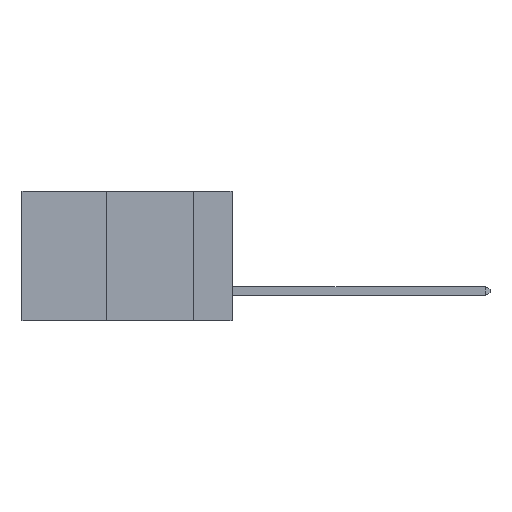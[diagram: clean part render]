
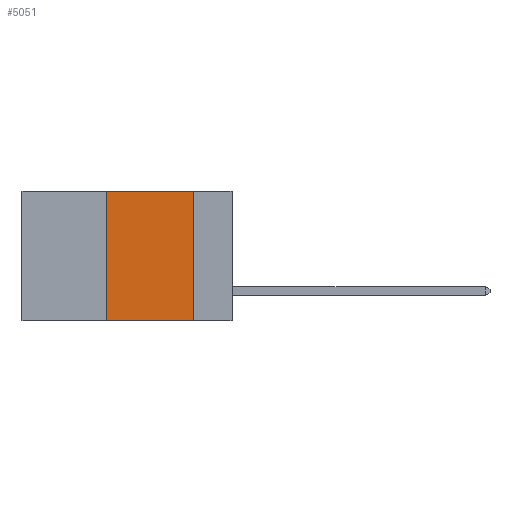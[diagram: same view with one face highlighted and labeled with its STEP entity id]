
A CAD part, left-side view. The second image highlights one B-rep face of the part: STEP entity #5051.
In plain terms, the highlighted planar face has unit normal (-1, 0, 0).
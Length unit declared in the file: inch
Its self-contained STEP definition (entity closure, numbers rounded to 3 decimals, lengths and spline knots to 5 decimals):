
#315 = ORIENTED_EDGE ( 'NONE', *, *, #6782, .F. ) ;
#455 = VECTOR ( 'NONE', #13491, 39.37008 ) ;
#505 = ORIENTED_EDGE ( 'NONE', *, *, #12875, .T. ) ;
#1597 = CARTESIAN_POINT ( 'NONE',  ( 0., 0.11, 0. ) ) ;
#2081 = CARTESIAN_POINT ( 'NONE',  ( 0., 0.6, 0. ) ) ;
#2132 = DIRECTION ( 'NONE',  ( 0., -1., 0. ) ) ;
#2200 = EDGE_CURVE ( 'NONE', #9139, #2787, #4364, .T. ) ;
#2245 = ORIENTED_EDGE ( 'NONE', *, *, #2200, .F. ) ;
#2416 = DIRECTION ( 'NONE',  ( 0., 0., 1. ) ) ;
#2787 = VERTEX_POINT ( 'NONE', #1597 ) ;
#3052 = CARTESIAN_POINT ( 'NONE',  ( 0., 0.6, 0. ) ) ;
#3167 = CARTESIAN_POINT ( 'NONE',  ( 0., 0.36, 0. ) ) ;
#3324 = PLANE ( 'NONE',  #12195 ) ;
#3419 = ORIENTED_EDGE ( 'NONE', *, *, #7545, .F. ) ;
#3563 = DIRECTION ( 'NONE',  ( 1., 0., 0. ) ) ;
#3564 = DIRECTION ( 'NONE',  ( 0., 0., -1. ) ) ;
#4044 = VECTOR ( 'NONE', #7032, 39.37008 ) ;
#4364 = LINE ( 'NONE', #2081, #9705 ) ;
#5051 = ADVANCED_FACE ( 'NONE', ( #11603 ), #3324, .F. ) ;
#5469 = CARTESIAN_POINT ( 'NONE',  ( 0., 0.6, -0.37 ) ) ;
#6782 = EDGE_CURVE ( 'NONE', #10463, #9139, #8348, .T. ) ;
#7032 = DIRECTION ( 'NONE',  ( 0., 0., -1. ) ) ;
#7115 = CARTESIAN_POINT ( 'NONE',  ( 0., 0.36, -0.37 ) ) ;
#7545 = EDGE_CURVE ( 'NONE', #2787, #11419, #9720, .T. ) ;
#8348 = LINE ( 'NONE', #8963, #13176 ) ;
#8963 = CARTESIAN_POINT ( 'NONE',  ( 0., 0.36, 0. ) ) ;
#9139 = VERTEX_POINT ( 'NONE', #3167 ) ;
#9197 = EDGE_LOOP ( 'NONE', ( #3419, #2245, #315, #505 ) ) ;
#9705 = VECTOR ( 'NONE', #2132, 39.37008 ) ;
#9720 = LINE ( 'NONE', #12977, #4044 ) ;
#10463 = VERTEX_POINT ( 'NONE', #7115 ) ;
#11419 = VERTEX_POINT ( 'NONE', #11716 ) ;
#11603 = FACE_OUTER_BOUND ( 'NONE', #9197, .T. ) ;
#11716 = CARTESIAN_POINT ( 'NONE',  ( 0., 0.11, -0.37 ) ) ;
#11856 = LINE ( 'NONE', #5469, #455 ) ;
#12195 = AXIS2_PLACEMENT_3D ( 'NONE', #3052, #3563, #3564 ) ;
#12875 = EDGE_CURVE ( 'NONE', #10463, #11419, #11856, .T. ) ;
#12977 = CARTESIAN_POINT ( 'NONE',  ( 0., 0.11, 0. ) ) ;
#13176 = VECTOR ( 'NONE', #2416, 39.37008 ) ;
#13491 = DIRECTION ( 'NONE',  ( 0., -1., 0. ) ) ;
